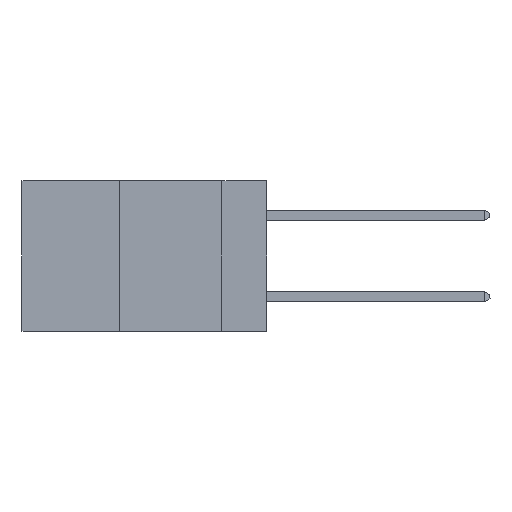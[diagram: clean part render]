
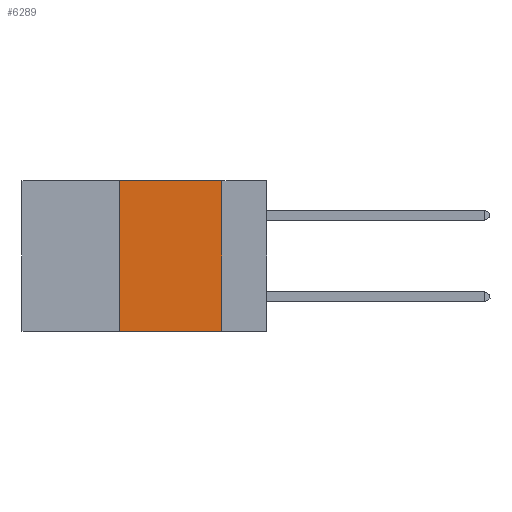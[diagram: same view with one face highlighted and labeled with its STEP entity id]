
A CAD part, left-side view. The second image highlights one B-rep face of the part: STEP entity #6289.
In plain terms, the highlighted planar face has unit normal (-1, 0, 0).
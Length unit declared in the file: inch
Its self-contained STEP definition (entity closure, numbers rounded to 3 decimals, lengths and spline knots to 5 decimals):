
#129 = LINE ( 'NONE', #1689, #9329 ) ;
#890 = EDGE_CURVE ( 'NONE', #8194, #4934, #1737, .T. ) ;
#1015 = DIRECTION ( 'NONE',  ( 0., 0., -1. ) ) ;
#1319 = ORIENTED_EDGE ( 'NONE', *, *, #6073, .F. ) ;
#1689 = CARTESIAN_POINT ( 'NONE',  ( 0., 0.36, 0. ) ) ;
#1737 = LINE ( 'NONE', #7954, #9864 ) ;
#2250 = AXIS2_PLACEMENT_3D ( 'NONE', #10416, #6031, #3476 ) ;
#2378 = LINE ( 'NONE', #10299, #2526 ) ;
#2526 = VECTOR ( 'NONE', #5955, 39.37008 ) ;
#2648 = DIRECTION ( 'NONE',  ( 0., -1., 0. ) ) ;
#2949 = CARTESIAN_POINT ( 'NONE',  ( 0., 0.11, 0. ) ) ;
#3242 = FACE_OUTER_BOUND ( 'NONE', #8896, .T. ) ;
#3376 = VERTEX_POINT ( 'NONE', #4564 ) ;
#3446 = EDGE_CURVE ( 'NONE', #5664, #4934, #4007, .T. ) ;
#3476 = DIRECTION ( 'NONE',  ( 0., 0., -1. ) ) ;
#4007 = LINE ( 'NONE', #5521, #9979 ) ;
#4213 = PLANE ( 'NONE',  #2250 ) ;
#4347 = CARTESIAN_POINT ( 'NONE',  ( 0., 0.36, -0.37 ) ) ;
#4564 = CARTESIAN_POINT ( 'NONE',  ( 0., 0.36, 0. ) ) ;
#4933 = CARTESIAN_POINT ( 'NONE',  ( 0., 0.11, -0.37 ) ) ;
#4934 = VERTEX_POINT ( 'NONE', #4933 ) ;
#5521 = CARTESIAN_POINT ( 'NONE',  ( 0., 0.11, 0. ) ) ;
#5664 = VERTEX_POINT ( 'NONE', #2949 ) ;
#5955 = DIRECTION ( 'NONE',  ( 0., -1., 0. ) ) ;
#6031 = DIRECTION ( 'NONE',  ( 1., 0., 0. ) ) ;
#6073 = EDGE_CURVE ( 'NONE', #8194, #3376, #129, .T. ) ;
#6289 = ADVANCED_FACE ( 'NONE', ( #3242 ), #4213, .F. ) ;
#6307 = DIRECTION ( 'NONE',  ( 0., 0., 1. ) ) ;
#6444 = EDGE_CURVE ( 'NONE', #3376, #5664, #2378, .T. ) ;
#7954 = CARTESIAN_POINT ( 'NONE',  ( 0., 0.6, -0.37 ) ) ;
#8194 = VERTEX_POINT ( 'NONE', #4347 ) ;
#8426 = ORIENTED_EDGE ( 'NONE', *, *, #3446, .F. ) ;
#8896 = EDGE_LOOP ( 'NONE', ( #8426, #8972, #1319, #10398 ) ) ;
#8972 = ORIENTED_EDGE ( 'NONE', *, *, #6444, .F. ) ;
#9329 = VECTOR ( 'NONE', #6307, 39.37008 ) ;
#9864 = VECTOR ( 'NONE', #2648, 39.37008 ) ;
#9979 = VECTOR ( 'NONE', #1015, 39.37008 ) ;
#10299 = CARTESIAN_POINT ( 'NONE',  ( 0., 0.6, 0. ) ) ;
#10398 = ORIENTED_EDGE ( 'NONE', *, *, #890, .T. ) ;
#10416 = CARTESIAN_POINT ( 'NONE',  ( 0., 0.6, 0. ) ) ;
